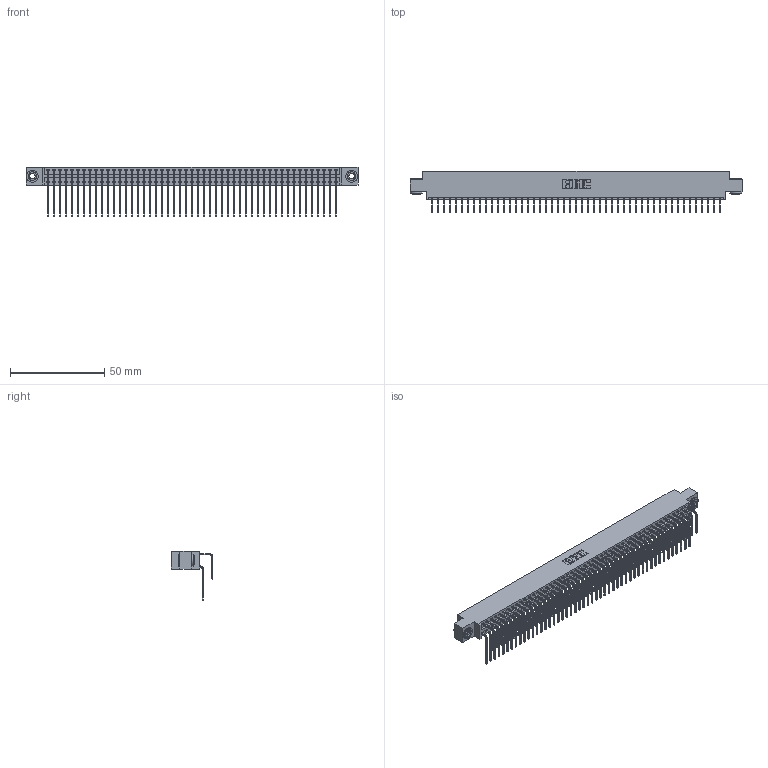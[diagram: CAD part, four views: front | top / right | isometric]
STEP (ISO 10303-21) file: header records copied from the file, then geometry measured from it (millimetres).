
FILE_DESCRIPTION (( 'STEP AP203' ), '1' );
FILE_NAME ('346-098-558-803.STEP', '2018-08-30T09:35:24', ( '' ), ( '' ), 'SwSTEP 2.0', 'SolidWorks 2016', '' );
FILE_SCHEMA (( 'CONFIG_CONTROL_DESIGN' ));
Length unit declared in the file: inch
Products named in the file (5): 345-292-001_558 559 Tail - 1; 345-292-001_558 Tail - 2; 345-250-002_345-250-002-102; 346-098-558-803; 346 Part_0.170 Offset - 0.156 Dia-TH
Assembly tree (101 placements, depth 2):
  346-098-558-803
    346 Part_0.170 Offset - 0.156 Dia-TH
    345-292-001_558 559 Tail - 1  x49
    345-292-001_558 Tail - 2  x49
    345-250-002_345-250-002-102  x2
Bounding box: 176.15 x 22.16 x 26.16 mm (x, y, z)
Volume: 17661.2 mm3; surface area: 27492.4 mm2
Topology: 101 solids, 101 shells, 5456 faces, 16195 edges, 10662 vertices
Faces by surface type: plane 3716, cylinder 1732, cone 8
Entity records: 33602 total; most frequent: CARTESIAN_POINT 5558, ORIENTED_EDGE 5434, DIRECTION 4951, EDGE_CURVE 2717, VECTOR 2325, LINE 2325, VERTEX_POINT 1806, AXIS2_PLACEMENT_3D 1313
